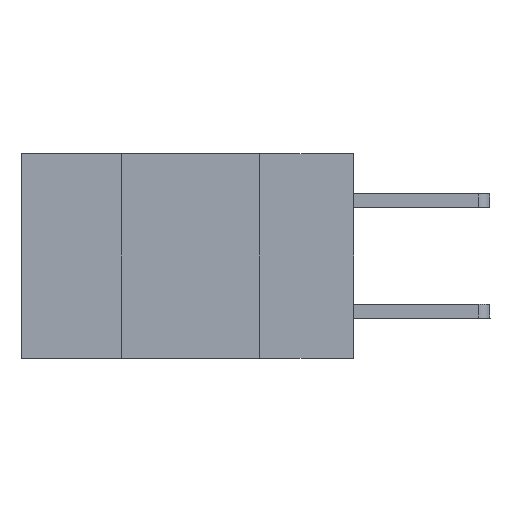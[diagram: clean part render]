
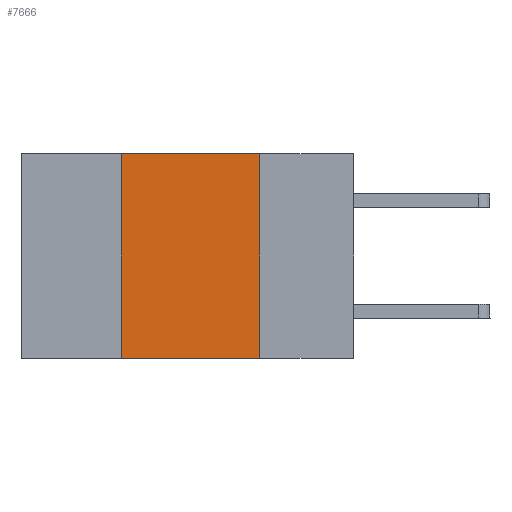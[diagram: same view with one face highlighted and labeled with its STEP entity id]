
A CAD part, left-side view. The second image highlights one B-rep face of the part: STEP entity #7666.
In plain terms, the highlighted planar face has unit normal (-1, 0, 0).
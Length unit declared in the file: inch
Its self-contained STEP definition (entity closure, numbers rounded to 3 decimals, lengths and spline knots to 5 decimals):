
#159 = CARTESIAN_POINT ( 'NONE',  ( 0., 0.42, -0.37 ) ) ;
#1332 = ORIENTED_EDGE ( 'NONE', *, *, #2149, .F. ) ;
#1838 = VERTEX_POINT ( 'NONE', #8982 ) ;
#1839 = DIRECTION ( 'NONE',  ( 0., 0., 1. ) ) ;
#2149 = EDGE_CURVE ( 'NONE', #1838, #7662, #11872, .T. ) ;
#2227 = VECTOR ( 'NONE', #4387, 39.37008 ) ;
#2410 = EDGE_CURVE ( 'NONE', #7662, #12520, #3168, .T. ) ;
#2723 = EDGE_LOOP ( 'NONE', ( #12838, #1332, #10842, #5128 ) ) ;
#2866 = CARTESIAN_POINT ( 'NONE',  ( 0., 0.17, -0.37 ) ) ;
#2944 = DIRECTION ( 'NONE',  ( 1., 0., 0. ) ) ;
#3168 = LINE ( 'NONE', #7031, #10016 ) ;
#3790 = VECTOR ( 'NONE', #6123, 39.37008 ) ;
#4387 = DIRECTION ( 'NONE',  ( 0., -1., 0. ) ) ;
#4807 = EDGE_CURVE ( 'NONE', #5991, #1838, #7442, .T. ) ;
#5009 = VECTOR ( 'NONE', #1839, 39.37008 ) ;
#5128 = ORIENTED_EDGE ( 'NONE', *, *, #14263, .T. ) ;
#5192 = FACE_OUTER_BOUND ( 'NONE', #2723, .T. ) ;
#5991 = VERTEX_POINT ( 'NONE', #159 ) ;
#6123 = DIRECTION ( 'NONE',  ( 0., -1., 0. ) ) ;
#6463 = CARTESIAN_POINT ( 'NONE',  ( 0., 0.42, 0. ) ) ;
#6884 = DIRECTION ( 'NONE',  ( 0., 0., -1. ) ) ;
#7031 = CARTESIAN_POINT ( 'NONE',  ( 0., 0.17, 0. ) ) ;
#7241 = CARTESIAN_POINT ( 'NONE',  ( 0., 0.6, 0. ) ) ;
#7433 = CARTESIAN_POINT ( 'NONE',  ( 0., 0.17, 0. ) ) ;
#7442 = LINE ( 'NONE', #6463, #5009 ) ;
#7662 = VERTEX_POINT ( 'NONE', #7433 ) ;
#7666 = ADVANCED_FACE ( 'NONE', ( #5192 ), #13163, .F. ) ;
#7969 = LINE ( 'NONE', #12580, #2227 ) ;
#8982 = CARTESIAN_POINT ( 'NONE',  ( 0., 0.42, 0. ) ) ;
#9615 = AXIS2_PLACEMENT_3D ( 'NONE', #13304, #2944, #10866 ) ;
#10016 = VECTOR ( 'NONE', #6884, 39.37008 ) ;
#10842 = ORIENTED_EDGE ( 'NONE', *, *, #4807, .F. ) ;
#10866 = DIRECTION ( 'NONE',  ( 0., 0., -1. ) ) ;
#11872 = LINE ( 'NONE', #7241, #3790 ) ;
#12520 = VERTEX_POINT ( 'NONE', #2866 ) ;
#12580 = CARTESIAN_POINT ( 'NONE',  ( 0., 0.6, -0.37 ) ) ;
#12838 = ORIENTED_EDGE ( 'NONE', *, *, #2410, .F. ) ;
#13163 = PLANE ( 'NONE',  #9615 ) ;
#13304 = CARTESIAN_POINT ( 'NONE',  ( 0., 0.6, 0. ) ) ;
#14263 = EDGE_CURVE ( 'NONE', #5991, #12520, #7969, .T. ) ;
